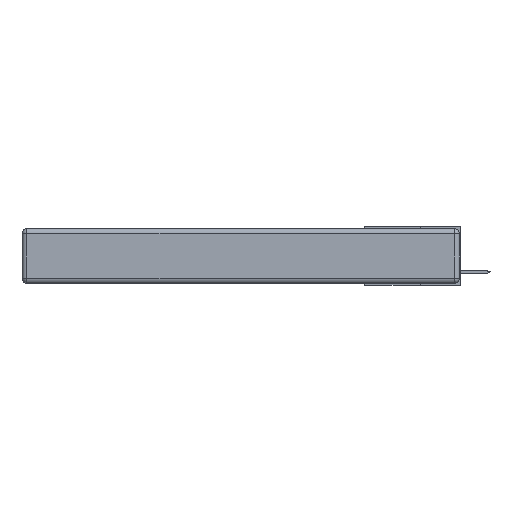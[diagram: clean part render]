
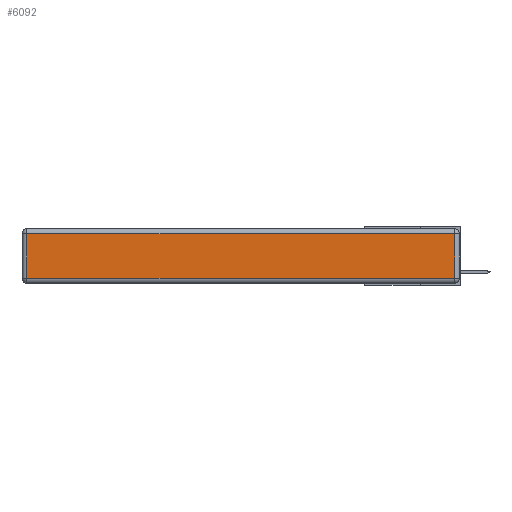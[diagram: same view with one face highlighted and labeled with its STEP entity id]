
A CAD part, left-side view. The second image highlights one B-rep face of the part: STEP entity #6092.
In plain terms, the highlighted planar face has unit normal (-1, 0, 0).
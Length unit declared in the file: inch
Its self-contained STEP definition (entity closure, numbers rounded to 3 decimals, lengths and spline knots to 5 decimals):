
#313 = LINE ( 'NONE', #5962, #3742 ) ;
#548 = CARTESIAN_POINT ( 'NONE',  ( 0., 2.72, -0.03 ) ) ;
#641 = DIRECTION ( 'NONE',  ( 0., -1., 0. ) ) ;
#994 = CARTESIAN_POINT ( 'NONE',  ( 0., 0.03, -0.313 ) ) ;
#1490 = VERTEX_POINT ( 'NONE', #12918 ) ;
#2361 = DIRECTION ( 'NONE',  ( 0., 0., 1. ) ) ;
#2565 = VERTEX_POINT ( 'NONE', #548 ) ;
#3023 = VECTOR ( 'NONE', #7025, 39.37008 ) ;
#3742 = VECTOR ( 'NONE', #2361, 39.37008 ) ;
#4135 = DIRECTION ( 'NONE',  ( -1., 0., 0. ) ) ;
#4150 = ORIENTED_EDGE ( 'NONE', *, *, #7568, .T. ) ;
#4842 = VECTOR ( 'NONE', #11081, 39.37008 ) ;
#5962 = CARTESIAN_POINT ( 'NONE',  ( 0., 0.03, -0.343 ) ) ;
#6092 = ADVANCED_FACE ( 'NONE', ( #10079 ), #13649, .T. ) ;
#6498 = CARTESIAN_POINT ( 'NONE',  ( 0., 0., -0.313 ) ) ;
#7015 = VERTEX_POINT ( 'NONE', #994 ) ;
#7025 = DIRECTION ( 'NONE',  ( 0., 1., 0. ) ) ;
#7568 = EDGE_CURVE ( 'NONE', #1490, #2565, #15312, .T. ) ;
#7785 = EDGE_CURVE ( 'NONE', #7015, #1490, #313, .T. ) ;
#7980 = ORIENTED_EDGE ( 'NONE', *, *, #7785, .T. ) ;
#8439 = LINE ( 'NONE', #9684, #4842 ) ;
#9684 = CARTESIAN_POINT ( 'NONE',  ( 0., 2.72, -0.343 ) ) ;
#9785 = AXIS2_PLACEMENT_3D ( 'NONE', #12644, #4135, #11262 ) ;
#10079 = FACE_OUTER_BOUND ( 'NONE', #11239, .T. ) ;
#10201 = CARTESIAN_POINT ( 'NONE',  ( 0., 2.72, -0.313 ) ) ;
#10640 = EDGE_CURVE ( 'NONE', #2565, #10954, #8439, .T. ) ;
#10954 = VERTEX_POINT ( 'NONE', #10201 ) ;
#10972 = ORIENTED_EDGE ( 'NONE', *, *, #10640, .T. ) ;
#11081 = DIRECTION ( 'NONE',  ( 0., 0., -1. ) ) ;
#11239 = EDGE_LOOP ( 'NONE', ( #13600, #7980, #4150, #10972 ) ) ;
#11262 = DIRECTION ( 'NONE',  ( 0., 0., 1. ) ) ;
#12074 = VECTOR ( 'NONE', #641, 39.37008 ) ;
#12644 = CARTESIAN_POINT ( 'NONE',  ( 0., 0., -0.343 ) ) ;
#12918 = CARTESIAN_POINT ( 'NONE',  ( 0., 0.03, -0.03 ) ) ;
#12950 = CARTESIAN_POINT ( 'NONE',  ( 0., 2.75, -0.03 ) ) ;
#13371 = LINE ( 'NONE', #6498, #12074 ) ;
#13600 = ORIENTED_EDGE ( 'NONE', *, *, #13995, .T. ) ;
#13649 = PLANE ( 'NONE',  #9785 ) ;
#13995 = EDGE_CURVE ( 'NONE', #10954, #7015, #13371, .T. ) ;
#15312 = LINE ( 'NONE', #12950, #3023 ) ;
